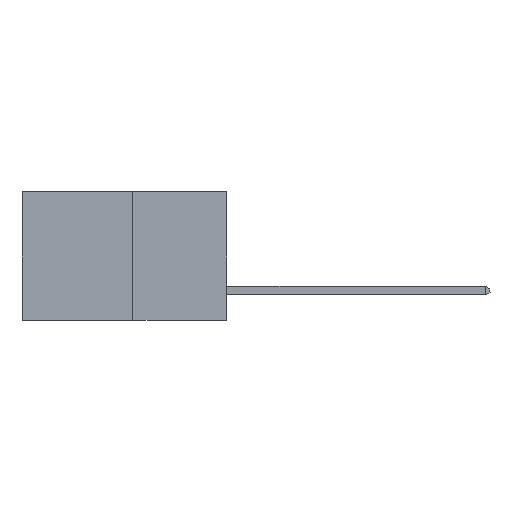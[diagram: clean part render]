
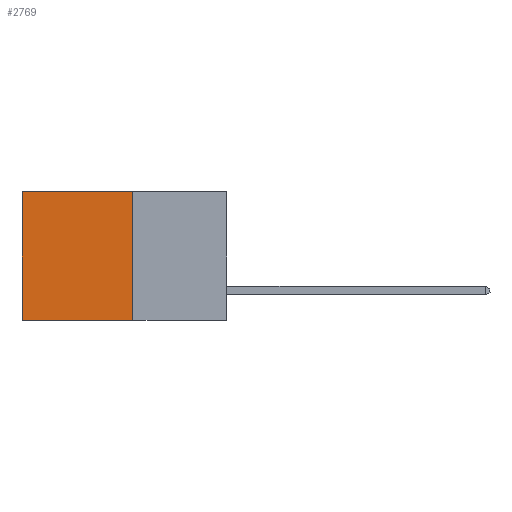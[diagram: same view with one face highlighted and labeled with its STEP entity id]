
A CAD part, left-side view. The second image highlights one B-rep face of the part: STEP entity #2769.
In plain terms, the highlighted planar face has unit normal (-1, 0, 0).
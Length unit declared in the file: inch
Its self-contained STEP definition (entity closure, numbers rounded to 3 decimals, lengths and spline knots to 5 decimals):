
#17 = CARTESIAN_POINT ( 'NONE',  ( 0.277, 0.59, -0.37 ) ) ;
#657 = EDGE_CURVE ( 'NONE', #10312, #5237, #10507, .T. ) ;
#1091 = VERTEX_POINT ( 'NONE', #4985 ) ;
#1164 = CARTESIAN_POINT ( 'NONE',  ( 0.277, 0.59, -0.37 ) ) ;
#1605 = VECTOR ( 'NONE', #8673, 39.37008 ) ;
#1676 = EDGE_CURVE ( 'NONE', #1091, #2441, #8362, .T. ) ;
#1917 = DIRECTION ( 'NONE',  ( 0., 0., -1. ) ) ;
#2295 = EDGE_LOOP ( 'NONE', ( #5195, #5148, #5070, #5032 ) ) ;
#2441 = VERTEX_POINT ( 'NONE', #1164 ) ;
#2769 = ADVANCED_FACE ( 'NONE', ( #8666 ), #6420, .F. ) ;
#4215 = CARTESIAN_POINT ( 'NONE',  ( 0.277, 0.27, -0.37 ) ) ;
#4866 = DIRECTION ( 'NONE',  ( 0., 0., -1. ) ) ;
#4985 = CARTESIAN_POINT ( 'NONE',  ( 0.277, 0.59, 0. ) ) ;
#5032 = ORIENTED_EDGE ( 'NONE', *, *, #6683, .T. ) ;
#5070 = ORIENTED_EDGE ( 'NONE', *, *, #657, .F. ) ;
#5138 = EDGE_CURVE ( 'NONE', #5237, #2441, #5377, .T. ) ;
#5148 = ORIENTED_EDGE ( 'NONE', *, *, #5138, .F. ) ;
#5195 = ORIENTED_EDGE ( 'NONE', *, *, #1676, .T. ) ;
#5237 = VERTEX_POINT ( 'NONE', #6311 ) ;
#5377 = LINE ( 'NONE', #8504, #5642 ) ;
#5642 = VECTOR ( 'NONE', #8370, 39.37008 ) ;
#5895 = CARTESIAN_POINT ( 'NONE',  ( 0.277, 0.27, 0. ) ) ;
#5937 = DIRECTION ( 'NONE',  ( 1., 0., 0. ) ) ;
#6311 = CARTESIAN_POINT ( 'NONE',  ( 0.277, 0.27, -0.37 ) ) ;
#6420 = PLANE ( 'NONE',  #9052 ) ;
#6683 = EDGE_CURVE ( 'NONE', #10312, #1091, #9995, .T. ) ;
#7862 = CARTESIAN_POINT ( 'NONE',  ( 0.277, 0.27, -0.37 ) ) ;
#8362 = LINE ( 'NONE', #17, #1605 ) ;
#8370 = DIRECTION ( 'NONE',  ( 0., 1., 0. ) ) ;
#8504 = CARTESIAN_POINT ( 'NONE',  ( 0.277, 0.27, -0.37 ) ) ;
#8666 = FACE_OUTER_BOUND ( 'NONE', #2295, .T. ) ;
#8673 = DIRECTION ( 'NONE',  ( 0., 0., -1. ) ) ;
#9052 = AXIS2_PLACEMENT_3D ( 'NONE', #7862, #5937, #4866 ) ;
#9285 = CARTESIAN_POINT ( 'NONE',  ( 0.277, 0.27, 0. ) ) ;
#9995 = LINE ( 'NONE', #5895, #10662 ) ;
#10069 = VECTOR ( 'NONE', #1917, 39.37008 ) ;
#10312 = VERTEX_POINT ( 'NONE', #9285 ) ;
#10486 = DIRECTION ( 'NONE',  ( 0., 1., 0. ) ) ;
#10507 = LINE ( 'NONE', #4215, #10069 ) ;
#10662 = VECTOR ( 'NONE', #10486, 39.37008 ) ;
